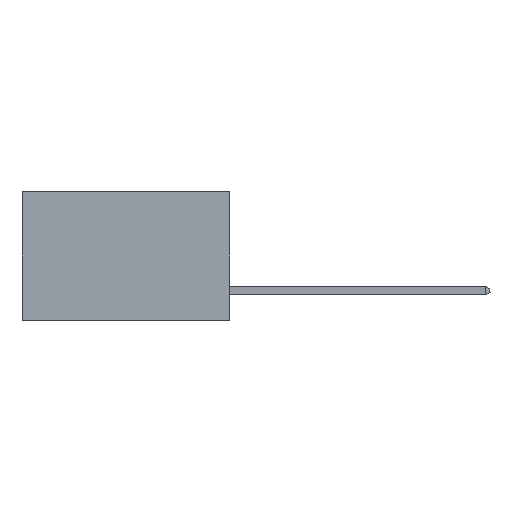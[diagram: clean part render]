
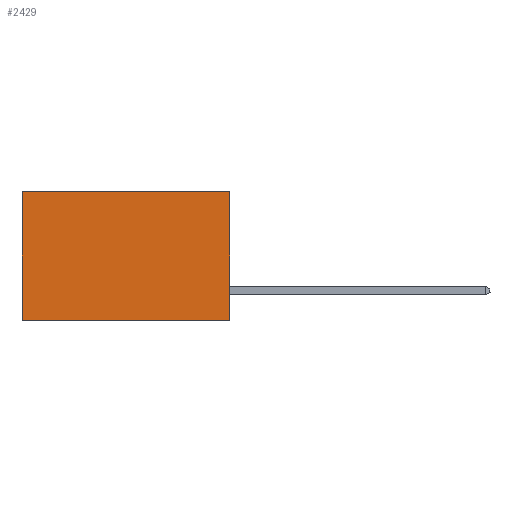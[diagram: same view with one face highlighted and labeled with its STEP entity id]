
A CAD part, left-side view. The second image highlights one B-rep face of the part: STEP entity #2429.
In plain terms, the highlighted planar face has unit normal (-1, 0, 0).
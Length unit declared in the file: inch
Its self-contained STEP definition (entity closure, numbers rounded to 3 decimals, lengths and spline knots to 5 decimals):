
#558 = VERTEX_POINT ( 'NONE', #3831 ) ;
#1139 = EDGE_CURVE ( 'NONE', #558, #1361, #25488, .T. ) ;
#1313 = CARTESIAN_POINT ( 'NONE',  ( 0.298, 0., 0. ) ) ;
#1361 = VERTEX_POINT ( 'NONE', #17588 ) ;
#1927 = VECTOR ( 'NONE', #3825, 39.37008 ) ;
#2306 = LINE ( 'NONE', #22593, #23502 ) ;
#2429 = ADVANCED_FACE ( 'NONE', ( #16995 ), #5944, .F. ) ;
#2523 = LINE ( 'NONE', #1313, #22439 ) ;
#2598 = EDGE_LOOP ( 'NONE', ( #19817, #22147, #24644, #14998 ) ) ;
#3825 = DIRECTION ( 'NONE',  ( 0., 0., -1. ) ) ;
#3831 = CARTESIAN_POINT ( 'NONE',  ( 0.298, 0., 0. ) ) ;
#5944 = PLANE ( 'NONE',  #9721 ) ;
#6659 = CARTESIAN_POINT ( 'NONE',  ( 0.298, 0., 0. ) ) ;
#7395 = DIRECTION ( 'NONE',  ( 0., 0., -1. ) ) ;
#8857 = CARTESIAN_POINT ( 'NONE',  ( 0.298, 0.6, -0.37 ) ) ;
#9051 = VECTOR ( 'NONE', #12419, 39.37008 ) ;
#9721 = AXIS2_PLACEMENT_3D ( 'NONE', #12019, #18146, #20309 ) ;
#11442 = EDGE_CURVE ( 'NONE', #12052, #26431, #2306, .T. ) ;
#12019 = CARTESIAN_POINT ( 'NONE',  ( 0.298, 0., 0. ) ) ;
#12052 = VERTEX_POINT ( 'NONE', #17757 ) ;
#12419 = DIRECTION ( 'NONE',  ( 0., 1., 0. ) ) ;
#14998 = ORIENTED_EDGE ( 'NONE', *, *, #1139, .T. ) ;
#16995 = FACE_OUTER_BOUND ( 'NONE', #2598, .T. ) ;
#17588 = CARTESIAN_POINT ( 'NONE',  ( 0.298, 0.6, 0. ) ) ;
#17757 = CARTESIAN_POINT ( 'NONE',  ( 0.298, 0., -0.37 ) ) ;
#18146 = DIRECTION ( 'NONE',  ( 1., 0., 0. ) ) ;
#18582 = LINE ( 'NONE', #24147, #1927 ) ;
#19817 = ORIENTED_EDGE ( 'NONE', *, *, #22306, .T. ) ;
#20309 = DIRECTION ( 'NONE',  ( 0., 0., -1. ) ) ;
#22147 = ORIENTED_EDGE ( 'NONE', *, *, #11442, .F. ) ;
#22306 = EDGE_CURVE ( 'NONE', #1361, #26431, #18582, .T. ) ;
#22428 = DIRECTION ( 'NONE',  ( 0., 1., 0. ) ) ;
#22439 = VECTOR ( 'NONE', #7395, 39.37008 ) ;
#22593 = CARTESIAN_POINT ( 'NONE',  ( 0.298, 0., -0.37 ) ) ;
#22854 = EDGE_CURVE ( 'NONE', #558, #12052, #2523, .T. ) ;
#23502 = VECTOR ( 'NONE', #22428, 39.37008 ) ;
#24147 = CARTESIAN_POINT ( 'NONE',  ( 0.298, 0.6, 0. ) ) ;
#24644 = ORIENTED_EDGE ( 'NONE', *, *, #22854, .F. ) ;
#25488 = LINE ( 'NONE', #6659, #9051 ) ;
#26431 = VERTEX_POINT ( 'NONE', #8857 ) ;
